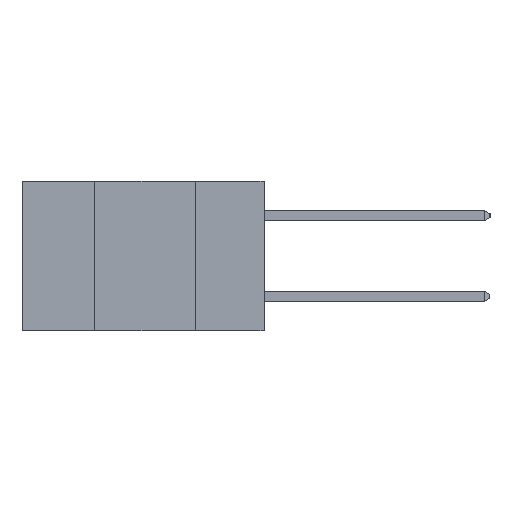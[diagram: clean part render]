
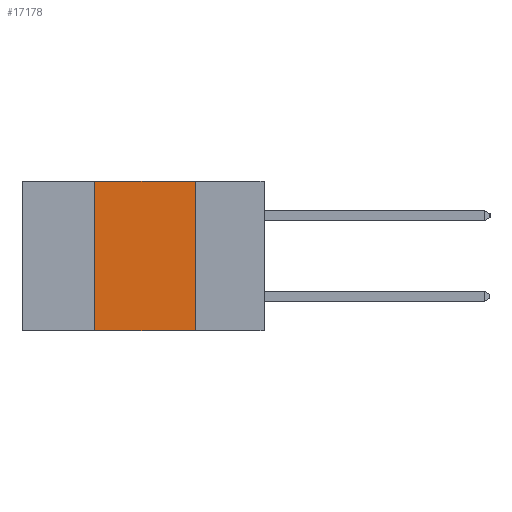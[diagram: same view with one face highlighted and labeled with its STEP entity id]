
A CAD part, left-side view. The second image highlights one B-rep face of the part: STEP entity #17178.
In plain terms, the highlighted planar face has unit normal (-1, 0, 0).
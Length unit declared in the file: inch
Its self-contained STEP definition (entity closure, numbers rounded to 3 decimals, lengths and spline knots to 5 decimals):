
#247 = VECTOR ( 'NONE', #14779, 39.37008 ) ;
#522 = ORIENTED_EDGE ( 'NONE', *, *, #7553, .F. ) ;
#652 = EDGE_CURVE ( 'NONE', #9372, #2160, #16592, .T. ) ;
#1123 = AXIS2_PLACEMENT_3D ( 'NONE', #4659, #4849, #7501 ) ;
#1483 = CARTESIAN_POINT ( 'NONE',  ( 0., 0.42, -0.37 ) ) ;
#2024 = ORIENTED_EDGE ( 'NONE', *, *, #5595, .F. ) ;
#2160 = VERTEX_POINT ( 'NONE', #8695 ) ;
#2402 = DIRECTION ( 'NONE',  ( 0., 0., 1. ) ) ;
#3517 = FACE_OUTER_BOUND ( 'NONE', #9985, .T. ) ;
#3647 = CARTESIAN_POINT ( 'NONE',  ( 0., 0.17, -0.37 ) ) ;
#4659 = CARTESIAN_POINT ( 'NONE',  ( 0., 0.6, 0. ) ) ;
#4849 = DIRECTION ( 'NONE',  ( 1., 0., 0. ) ) ;
#5071 = CARTESIAN_POINT ( 'NONE',  ( 0., 0.17, -0.37 ) ) ;
#5175 = CARTESIAN_POINT ( 'NONE',  ( 0., 0.42, 0. ) ) ;
#5232 = LINE ( 'NONE', #15913, #7222 ) ;
#5595 = EDGE_CURVE ( 'NONE', #2160, #11538, #14307, .T. ) ;
#5751 = DIRECTION ( 'NONE',  ( 0., -1., 0. ) ) ;
#7222 = VECTOR ( 'NONE', #2402, 39.37008 ) ;
#7501 = DIRECTION ( 'NONE',  ( 0., 0., -1. ) ) ;
#7553 = EDGE_CURVE ( 'NONE', #10432, #9372, #5232, .T. ) ;
#7893 = DIRECTION ( 'NONE',  ( 0., 0., -1. ) ) ;
#8695 = CARTESIAN_POINT ( 'NONE',  ( 0., 0.17, 0. ) ) ;
#9084 = VECTOR ( 'NONE', #7893, 39.37008 ) ;
#9372 = VERTEX_POINT ( 'NONE', #5175 ) ;
#9985 = EDGE_LOOP ( 'NONE', ( #2024, #14577, #522, #11210 ) ) ;
#10188 = EDGE_CURVE ( 'NONE', #10432, #11538, #13145, .T. ) ;
#10417 = CARTESIAN_POINT ( 'NONE',  ( 0., 0.6, -0.37 ) ) ;
#10432 = VERTEX_POINT ( 'NONE', #1483 ) ;
#11210 = ORIENTED_EDGE ( 'NONE', *, *, #10188, .T. ) ;
#11538 = VERTEX_POINT ( 'NONE', #3647 ) ;
#13145 = LINE ( 'NONE', #10417, #247 ) ;
#14307 = LINE ( 'NONE', #5071, #9084 ) ;
#14577 = ORIENTED_EDGE ( 'NONE', *, *, #652, .F. ) ;
#14662 = VECTOR ( 'NONE', #5751, 39.37008 ) ;
#14779 = DIRECTION ( 'NONE',  ( 0., -1., 0. ) ) ;
#15913 = CARTESIAN_POINT ( 'NONE',  ( 0., 0.42, -0.37 ) ) ;
#16330 = CARTESIAN_POINT ( 'NONE',  ( 0., 0.6, 0. ) ) ;
#16592 = LINE ( 'NONE', #16330, #14662 ) ;
#16830 = PLANE ( 'NONE',  #1123 ) ;
#17178 = ADVANCED_FACE ( 'NONE', ( #3517 ), #16830, .F. ) ;
